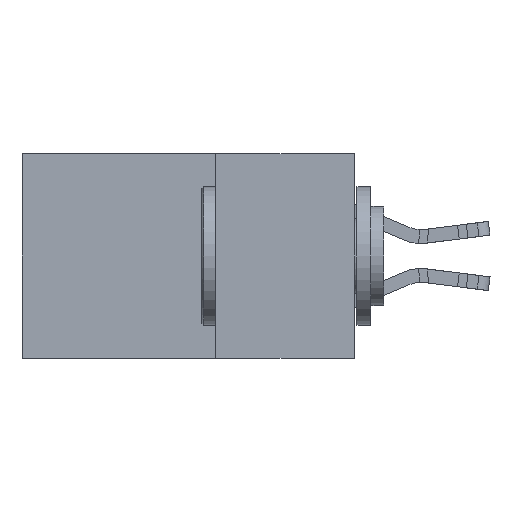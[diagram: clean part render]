
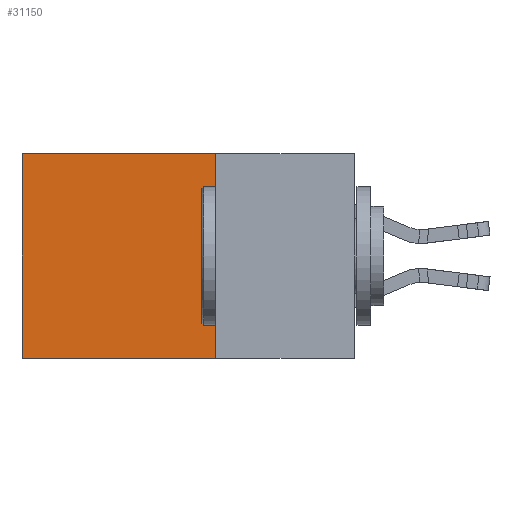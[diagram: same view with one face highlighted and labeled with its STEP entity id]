
A CAD part, left-side view. The second image highlights one B-rep face of the part: STEP entity #31150.
In plain terms, the highlighted planar face has unit normal (-1, 0, 0).
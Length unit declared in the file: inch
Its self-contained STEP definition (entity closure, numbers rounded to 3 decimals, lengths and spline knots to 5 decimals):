
#899 = VERTEX_POINT ( 'NONE', #18393 ) ;
#921 = CARTESIAN_POINT ( 'NONE',  ( 0.298, 0.25, 0. ) ) ;
#1410 = FACE_OUTER_BOUND ( 'NONE', #29416, .T. ) ;
#1980 = CARTESIAN_POINT ( 'NONE',  ( 0.298, 0.6, 0. ) ) ;
#2546 = LINE ( 'NONE', #14885, #3736 ) ;
#3437 = VERTEX_POINT ( 'NONE', #28812 ) ;
#3736 = VECTOR ( 'NONE', #32471, 39.37008 ) ;
#5465 = LINE ( 'NONE', #1980, #16229 ) ;
#6100 = VERTEX_POINT ( 'NONE', #20992 ) ;
#6710 = DIRECTION ( 'NONE',  ( 1., 0., 0. ) ) ;
#6861 = ORIENTED_EDGE ( 'NONE', *, *, #32581, .F. ) ;
#7526 = ORIENTED_EDGE ( 'NONE', *, *, #11208, .T. ) ;
#8694 = DIRECTION ( 'NONE',  ( 0., 1., 0. ) ) ;
#11208 = EDGE_CURVE ( 'NONE', #899, #6100, #27386, .T. ) ;
#11844 = LINE ( 'NONE', #14869, #30148 ) ;
#12208 = DIRECTION ( 'NONE',  ( 0., 0., -1. ) ) ;
#13979 = PLANE ( 'NONE',  #20534 ) ;
#14758 = DIRECTION ( 'NONE',  ( 0., 0., -1. ) ) ;
#14869 = CARTESIAN_POINT ( 'NONE',  ( 0.298, 0.25, 0. ) ) ;
#14885 = CARTESIAN_POINT ( 'NONE',  ( 0.298, 0.25, -0.37 ) ) ;
#16035 = CARTESIAN_POINT ( 'NONE',  ( 0.298, 0.6, -0.37 ) ) ;
#16229 = VECTOR ( 'NONE', #12208, 39.37008 ) ;
#18393 = CARTESIAN_POINT ( 'NONE',  ( 0.298, 0.25, 0. ) ) ;
#18781 = ORIENTED_EDGE ( 'NONE', *, *, #27607, .T. ) ;
#19419 = VECTOR ( 'NONE', #8694, 39.37008 ) ;
#20534 = AXIS2_PLACEMENT_3D ( 'NONE', #29652, #6710, #24512 ) ;
#20992 = CARTESIAN_POINT ( 'NONE',  ( 0.298, 0.6, 0. ) ) ;
#24512 = DIRECTION ( 'NONE',  ( 0., 0., -1. ) ) ;
#24655 = ORIENTED_EDGE ( 'NONE', *, *, #29268, .F. ) ;
#27386 = LINE ( 'NONE', #921, #19419 ) ;
#27607 = EDGE_CURVE ( 'NONE', #6100, #28407, #5465, .T. ) ;
#28407 = VERTEX_POINT ( 'NONE', #16035 ) ;
#28812 = CARTESIAN_POINT ( 'NONE',  ( 0.298, 0.25, -0.37 ) ) ;
#29268 = EDGE_CURVE ( 'NONE', #899, #3437, #11844, .T. ) ;
#29416 = EDGE_LOOP ( 'NONE', ( #18781, #6861, #24655, #7526 ) ) ;
#29652 = CARTESIAN_POINT ( 'NONE',  ( 0.298, 0.25, 0. ) ) ;
#30148 = VECTOR ( 'NONE', #14758, 39.37008 ) ;
#31150 = ADVANCED_FACE ( 'NONE', ( #1410 ), #13979, .F. ) ;
#32471 = DIRECTION ( 'NONE',  ( 0., 1., 0. ) ) ;
#32581 = EDGE_CURVE ( 'NONE', #3437, #28407, #2546, .T. ) ;
